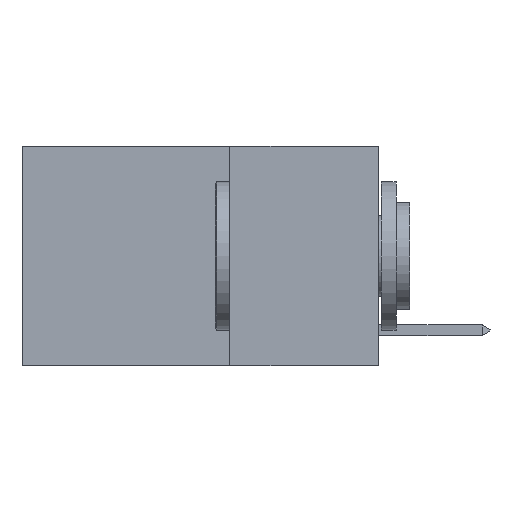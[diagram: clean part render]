
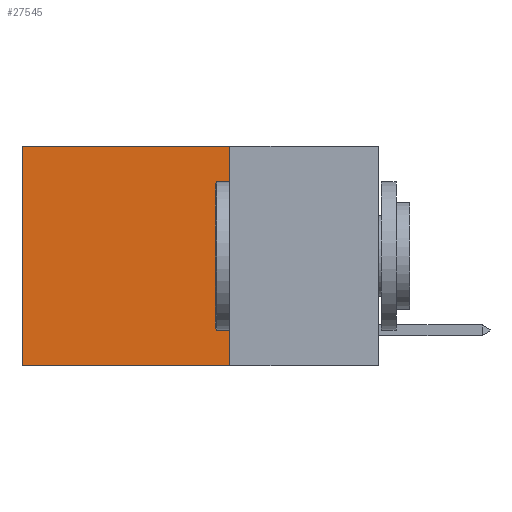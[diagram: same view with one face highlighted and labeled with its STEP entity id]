
A CAD part, left-side view. The second image highlights one B-rep face of the part: STEP entity #27545.
In plain terms, the highlighted planar face has unit normal (-1, 0, 0).
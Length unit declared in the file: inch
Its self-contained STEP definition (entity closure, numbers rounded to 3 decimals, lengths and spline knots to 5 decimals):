
#312 = EDGE_LOOP ( 'NONE', ( #19520, #19289, #15180, #5888 ) ) ;
#1188 = PLANE ( 'NONE',  #12835 ) ;
#1963 = VECTOR ( 'NONE', #13009, 39.37008 ) ;
#3082 = EDGE_CURVE ( 'NONE', #26196, #24054, #5326, .T. ) ;
#3567 = CARTESIAN_POINT ( 'NONE',  ( 0.2625, 0.25, 0. ) ) ;
#5326 = LINE ( 'NONE', #6455, #1963 ) ;
#5515 = CARTESIAN_POINT ( 'NONE',  ( 0.2625, 0.25, 0. ) ) ;
#5888 = ORIENTED_EDGE ( 'NONE', *, *, #8163, .T. ) ;
#6455 = CARTESIAN_POINT ( 'NONE',  ( 0.2625, 0.6, 0. ) ) ;
#7052 = LINE ( 'NONE', #15861, #17702 ) ;
#7580 = CARTESIAN_POINT ( 'NONE',  ( 0.2625, 0.6, -0.37 ) ) ;
#8163 = EDGE_CURVE ( 'NONE', #15032, #26196, #20797, .T. ) ;
#10311 = EDGE_CURVE ( 'NONE', #15032, #12901, #14542, .T. ) ;
#11055 = FACE_OUTER_BOUND ( 'NONE', #312, .T. ) ;
#11143 = CARTESIAN_POINT ( 'NONE',  ( 0.2625, 0.6, 0. ) ) ;
#12835 = AXIS2_PLACEMENT_3D ( 'NONE', #3567, #23036, #27332 ) ;
#12901 = VERTEX_POINT ( 'NONE', #21160 ) ;
#13009 = DIRECTION ( 'NONE',  ( 0., 0., -1. ) ) ;
#14542 = LINE ( 'NONE', #23391, #25488 ) ;
#15032 = VERTEX_POINT ( 'NONE', #27201 ) ;
#15180 = ORIENTED_EDGE ( 'NONE', *, *, #10311, .F. ) ;
#15861 = CARTESIAN_POINT ( 'NONE',  ( 0.2625, 0.25, -0.37 ) ) ;
#15967 = DIRECTION ( 'NONE',  ( 0., 1., 0. ) ) ;
#16598 = DIRECTION ( 'NONE',  ( 0., 1., 0. ) ) ;
#17702 = VECTOR ( 'NONE', #15967, 39.37008 ) ;
#19289 = ORIENTED_EDGE ( 'NONE', *, *, #20528, .F. ) ;
#19520 = ORIENTED_EDGE ( 'NONE', *, *, #3082, .T. ) ;
#20528 = EDGE_CURVE ( 'NONE', #12901, #24054, #7052, .T. ) ;
#20797 = LINE ( 'NONE', #5515, #27620 ) ;
#21160 = CARTESIAN_POINT ( 'NONE',  ( 0.2625, 0.25, -0.37 ) ) ;
#23036 = DIRECTION ( 'NONE',  ( 1., 0., 0. ) ) ;
#23391 = CARTESIAN_POINT ( 'NONE',  ( 0.2625, 0.25, 0. ) ) ;
#24054 = VERTEX_POINT ( 'NONE', #7580 ) ;
#25423 = DIRECTION ( 'NONE',  ( 0., 0., -1. ) ) ;
#25488 = VECTOR ( 'NONE', #25423, 39.37008 ) ;
#26196 = VERTEX_POINT ( 'NONE', #11143 ) ;
#27201 = CARTESIAN_POINT ( 'NONE',  ( 0.2625, 0.25, 0. ) ) ;
#27332 = DIRECTION ( 'NONE',  ( 0., 0., -1. ) ) ;
#27545 = ADVANCED_FACE ( 'NONE', ( #11055 ), #1188, .F. ) ;
#27620 = VECTOR ( 'NONE', #16598, 39.37008 ) ;
